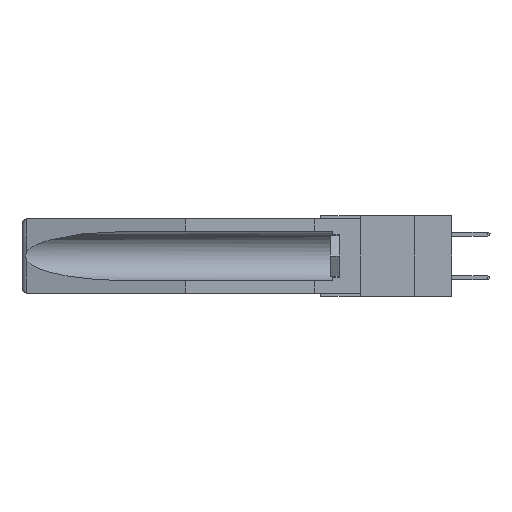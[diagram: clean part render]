
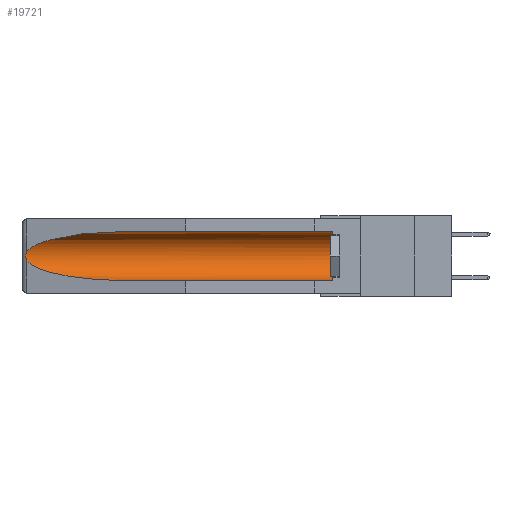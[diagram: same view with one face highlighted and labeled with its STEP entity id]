
A CAD part, left-side view. The second image highlights one B-rep face of the part: STEP entity #19721.
In plain terms, the highlighted cylindrical face has radius 2.857 mm (diameter 5.715 mm), a partial arc.
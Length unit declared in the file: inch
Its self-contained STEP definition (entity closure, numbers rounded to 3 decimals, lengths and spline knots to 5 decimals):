
#258 = EDGE_LOOP ( 'NONE', ( #29956, #5806, #31855, #12816, #27264, #8650 ) ) ;
#1090 = CARTESIAN_POINT ( 'NONE',  ( 0.2673, 1.53269, -0.17917 ) ) ;
#1588 = VERTEX_POINT ( 'NONE', #9800 ) ;
#1707 = CARTESIAN_POINT ( 'NONE',  ( 0.155, -0.30754, -0.284 ) ) ;
#2215 = VERTEX_POINT ( 'NONE', #29564 ) ;
#3450 = CARTESIAN_POINT ( 'NONE',  ( 0.26537, 1.52718, -0.19328 ) ) ;
#3672 = CARTESIAN_POINT ( 'NONE',  ( 0.2675, 1.53308, -0.17534 ) ) ;
#4157 = CARTESIAN_POINT ( 'NONE',  ( 0.26537, 1.52718, -0.19328 ) ) ;
#5463 = CARTESIAN_POINT ( 'NONE',  ( 0.26537, 1.52718, -0.14972 ) ) ;
#5565 = CARTESIAN_POINT ( 'NONE',  ( 0.155, 1.07973, -0.059 ) ) ;
#5568 = VERTEX_POINT ( 'NONE', #26044 ) ;
#5678 = VERTEX_POINT ( 'NONE', #10901 ) ;
#5806 = ORIENTED_EDGE ( 'NONE', *, *, #12791, .T. ) ;
#6203 = LINE ( 'NONE', #1707, #26735 ) ;
#8650 = ORIENTED_EDGE ( 'NONE', *, *, #12267, .T. ) ;
#9800 = CARTESIAN_POINT ( 'NONE',  ( 0.155, 0.126, -0.284 ) ) ;
#10116 = AXIS2_PLACEMENT_3D ( 'NONE', #21595, #15224, #27982 ) ;
#10271 = EDGE_CURVE ( 'NONE', #1588, #28367, #6203, .T. ) ;
#10901 = CARTESIAN_POINT ( 'NONE',  ( 0.26537, 1.52718, -0.19328 ) ) ;
#11897 = EDGE_CURVE ( 'NONE', #5568, #31992, #31849, .T. ) ;
#12267 = EDGE_CURVE ( 'NONE', #2215, #5568, #21602, .T. ) ;
#12385 = CARTESIAN_POINT ( 'NONE',  ( 0.155, -0.30754, -0.059 ) ) ;
#12791 = EDGE_CURVE ( 'NONE', #31992, #5678, #17009, .T. ) ;
#12816 = ORIENTED_EDGE ( 'NONE', *, *, #10271, .F. ) ;
#12821 = CARTESIAN_POINT ( 'NONE',  ( 0.25451, 1.48313, -0.09465 ) ) ;
#12928 = CARTESIAN_POINT ( 'NONE',  ( 0.155, 0.126, -0.1715 ) ) ;
#14897 = DIRECTION ( 'NONE',  ( 0., 1., 0. ) ) ;
#15105 = CYLINDRICAL_SURFACE ( 'NONE', #10116, 0.1125 ) ;
#15224 = DIRECTION ( 'NONE',  ( 0., 1., 0. ) ) ;
#16228 = CARTESIAN_POINT ( 'NONE',  ( 0.26537, 1.52718, -0.14972 ) ) ;
#16617 = CARTESIAN_POINT ( 'NONE',  ( 0.25451, 1.48313, -0.24835 ) ) ;
#16854 = AXIS2_PLACEMENT_3D ( 'NONE', #12928, #18104, #30204 ) ;
#17009 = B_SPLINE_CURVE_WITH_KNOTS ( 'NONE', 3,
 ( #18179, #20652, #25758, #20542, #28445, #3672, #1090, #23459, #30593, #3450 ),
 .UNSPECIFIED., .F., .F.,
 ( 4, 2, 2, 2, 4 ),
 ( 0., 0.00029, 0.00058, 0.00087, 0.00117 ),
 .UNSPECIFIED. ) ;
#18104 = DIRECTION ( 'NONE',  ( 0., -1., 0. ) ) ;
#18106 = CARTESIAN_POINT ( 'NONE',  ( 0.21114, 1.30732, -0.059 ) ) ;
#18179 = CARTESIAN_POINT ( 'NONE',  ( 0.26537, 1.52718, -0.14972 ) ) ;
#18940 = FACE_OUTER_BOUND ( 'NONE', #258, .T. ) ;
#19721 = ADVANCED_FACE ( 'NONE', ( #18940 ), #15105, .F. ) ;
#20358 =( BOUNDED_CURVE ( )  B_SPLINE_CURVE ( 3, ( #4157, #16617, #21347, #26448 ),
 .UNSPECIFIED., .F., .F. ) 
 B_SPLINE_CURVE_WITH_KNOTS ( ( 4, 4 ),
 ( 0.1948, 1.5708 ),
 .UNSPECIFIED. ) 
 CURVE ( )  GEOMETRIC_REPRESENTATION_ITEM ( )  RATIONAL_B_SPLINE_CURVE ( ( 1., 0.848, 0.848, 1. ) ) 
 REPRESENTATION_ITEM ( '' )  );
#20542 = CARTESIAN_POINT ( 'NONE',  ( 0.2673, 1.5327, -0.16383 ) ) ;
#20652 = CARTESIAN_POINT ( 'NONE',  ( 0.26597, 1.52961, -0.15275 ) ) ;
#21347 = CARTESIAN_POINT ( 'NONE',  ( 0.21114, 1.30732, -0.284 ) ) ;
#21595 = CARTESIAN_POINT ( 'NONE',  ( 0.155, -0.30754, -0.1715 ) ) ;
#21602 = LINE ( 'NONE', #12385, #30092 ) ;
#23459 = CARTESIAN_POINT ( 'NONE',  ( 0.26655, 1.53094, -0.18657 ) ) ;
#23900 = CARTESIAN_POINT ( 'NONE',  ( 0.155, 1.07973, -0.284 ) ) ;
#25758 = CARTESIAN_POINT ( 'NONE',  ( 0.26654, 1.53092, -0.15636 ) ) ;
#26044 = CARTESIAN_POINT ( 'NONE',  ( 0.155, 1.07973, -0.059 ) ) ;
#26189 = CIRCLE ( 'NONE', #16854, 0.1125 ) ;
#26297 = DIRECTION ( 'NONE',  ( 0., 1., 0. ) ) ;
#26389 = EDGE_CURVE ( 'NONE', #1588, #2215, #26189, .T. ) ;
#26448 = CARTESIAN_POINT ( 'NONE',  ( 0.155, 1.07973, -0.284 ) ) ;
#26735 = VECTOR ( 'NONE', #26297, 39.37008 ) ;
#27264 = ORIENTED_EDGE ( 'NONE', *, *, #26389, .T. ) ;
#27982 = DIRECTION ( 'NONE',  ( 0., 0., 1. ) ) ;
#28367 = VERTEX_POINT ( 'NONE', #23900 ) ;
#28445 = CARTESIAN_POINT ( 'NONE',  ( 0.2675, 1.53308, -0.16763 ) ) ;
#29267 = EDGE_CURVE ( 'NONE', #5678, #28367, #20358, .T. ) ;
#29564 = CARTESIAN_POINT ( 'NONE',  ( 0.155, 0.126, -0.059 ) ) ;
#29956 = ORIENTED_EDGE ( 'NONE', *, *, #11897, .T. ) ;
#30092 = VECTOR ( 'NONE', #14897, 39.37008 ) ;
#30204 = DIRECTION ( 'NONE',  ( 0., 0., 1. ) ) ;
#30593 = CARTESIAN_POINT ( 'NONE',  ( 0.26597, 1.5296, -0.19026 ) ) ;
#31849 =( BOUNDED_CURVE ( )  B_SPLINE_CURVE ( 3, ( #5565, #18106, #12821, #5463 ),
 .UNSPECIFIED., .F., .F. ) 
 B_SPLINE_CURVE_WITH_KNOTS ( ( 4, 4 ),
 ( 4.71239, 6.08839 ),
 .UNSPECIFIED. ) 
 CURVE ( )  GEOMETRIC_REPRESENTATION_ITEM ( )  RATIONAL_B_SPLINE_CURVE ( ( 1., 0.848, 0.848, 1. ) ) 
 REPRESENTATION_ITEM ( '' )  );
#31855 = ORIENTED_EDGE ( 'NONE', *, *, #29267, .T. ) ;
#31992 = VERTEX_POINT ( 'NONE', #16228 ) ;
